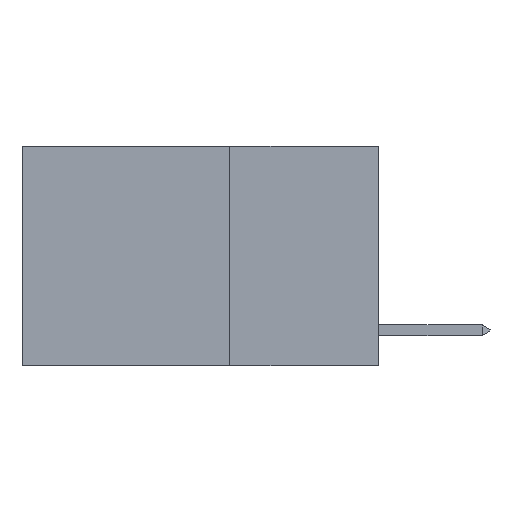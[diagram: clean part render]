
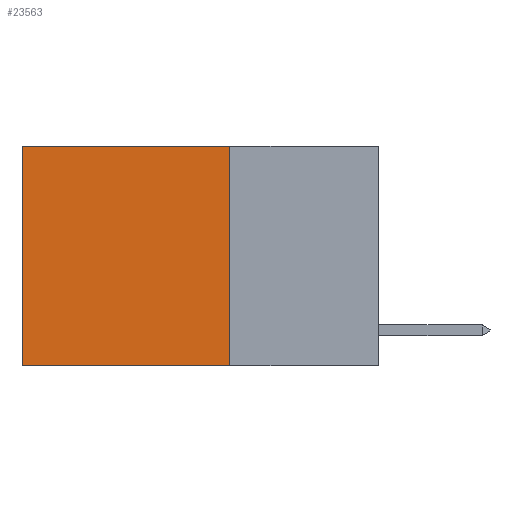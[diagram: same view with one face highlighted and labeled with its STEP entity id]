
A CAD part, left-side view. The second image highlights one B-rep face of the part: STEP entity #23563.
In plain terms, the highlighted planar face has unit normal (-1, 0, 0).
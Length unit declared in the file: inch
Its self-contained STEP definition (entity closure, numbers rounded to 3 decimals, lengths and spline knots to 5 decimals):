
#535 = CARTESIAN_POINT ( 'NONE',  ( 0.2625, 0.25, 0. ) ) ;
#2373 = EDGE_CURVE ( 'NONE', #26421, #4437, #10626, .T. ) ;
#2849 = CARTESIAN_POINT ( 'NONE',  ( 0.2625, 0.25, -0.37 ) ) ;
#3498 = EDGE_LOOP ( 'NONE', ( #3575, #3939, #6158, #15225 ) ) ;
#3575 = ORIENTED_EDGE ( 'NONE', *, *, #18750, .T. ) ;
#3939 = ORIENTED_EDGE ( 'NONE', *, *, #24286, .F. ) ;
#4083 = DIRECTION ( 'NONE',  ( 0., 0., -1. ) ) ;
#4437 = VERTEX_POINT ( 'NONE', #5912 ) ;
#5912 = CARTESIAN_POINT ( 'NONE',  ( 0.2625, 0.6, 0. ) ) ;
#6158 = ORIENTED_EDGE ( 'NONE', *, *, #18878, .F. ) ;
#6456 = LINE ( 'NONE', #19237, #13828 ) ;
#7098 = DIRECTION ( 'NONE',  ( 0., 1., 0. ) ) ;
#7802 = AXIS2_PLACEMENT_3D ( 'NONE', #12585, #19159, #4083 ) ;
#10568 = LINE ( 'NONE', #27316, #11898 ) ;
#10626 = LINE ( 'NONE', #19963, #16348 ) ;
#11476 = VECTOR ( 'NONE', #21646, 39.37008 ) ;
#11898 = VECTOR ( 'NONE', #19046, 39.37008 ) ;
#12150 = VERTEX_POINT ( 'NONE', #2849 ) ;
#12585 = CARTESIAN_POINT ( 'NONE',  ( 0.2625, 0.25, 0. ) ) ;
#13828 = VECTOR ( 'NONE', #19331, 39.37008 ) ;
#15225 = ORIENTED_EDGE ( 'NONE', *, *, #2373, .T. ) ;
#16348 = VECTOR ( 'NONE', #7098, 39.37008 ) ;
#17004 = CARTESIAN_POINT ( 'NONE',  ( 0.2625, 0.6, -0.37 ) ) ;
#18750 = EDGE_CURVE ( 'NONE', #4437, #23684, #6456, .T. ) ;
#18878 = EDGE_CURVE ( 'NONE', #26421, #12150, #21523, .T. ) ;
#19046 = DIRECTION ( 'NONE',  ( 0., 1., 0. ) ) ;
#19159 = DIRECTION ( 'NONE',  ( 1., 0., 0. ) ) ;
#19237 = CARTESIAN_POINT ( 'NONE',  ( 0.2625, 0.6, 0. ) ) ;
#19331 = DIRECTION ( 'NONE',  ( 0., 0., -1. ) ) ;
#19963 = CARTESIAN_POINT ( 'NONE',  ( 0.2625, 0.25, 0. ) ) ;
#20120 = CARTESIAN_POINT ( 'NONE',  ( 0.2625, 0.25, 0. ) ) ;
#21523 = LINE ( 'NONE', #535, #11476 ) ;
#21646 = DIRECTION ( 'NONE',  ( 0., 0., -1. ) ) ;
#23563 = ADVANCED_FACE ( 'NONE', ( #23802 ), #25558, .F. ) ;
#23684 = VERTEX_POINT ( 'NONE', #17004 ) ;
#23802 = FACE_OUTER_BOUND ( 'NONE', #3498, .T. ) ;
#24286 = EDGE_CURVE ( 'NONE', #12150, #23684, #10568, .T. ) ;
#25558 = PLANE ( 'NONE',  #7802 ) ;
#26421 = VERTEX_POINT ( 'NONE', #20120 ) ;
#27316 = CARTESIAN_POINT ( 'NONE',  ( 0.2625, 0.25, -0.37 ) ) ;
